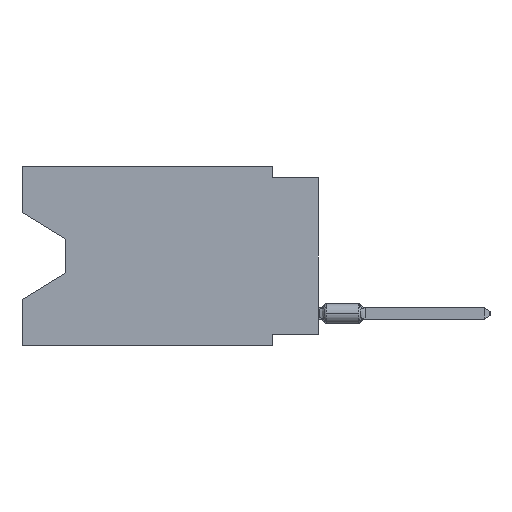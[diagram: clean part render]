
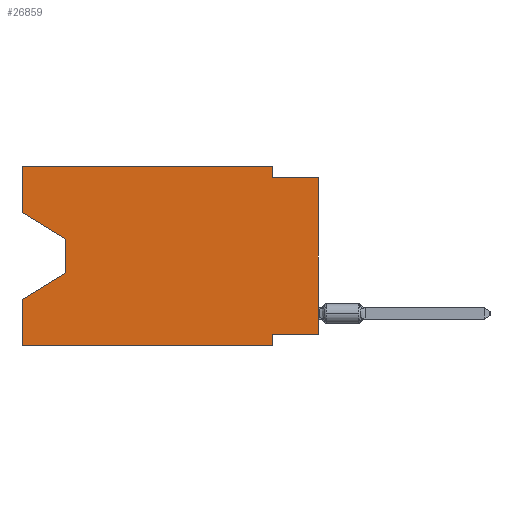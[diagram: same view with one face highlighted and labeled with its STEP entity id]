
A CAD part, left-side view. The second image highlights one B-rep face of the part: STEP entity #26859.
In plain terms, the highlighted planar face has unit normal (-1, 0, 0).
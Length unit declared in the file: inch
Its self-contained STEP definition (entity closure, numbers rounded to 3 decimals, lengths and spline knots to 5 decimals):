
#776 = CARTESIAN_POINT ( 'NONE',  ( 0., 0., -0.365 ) ) ;
#934 = LINE ( 'NONE', #68557, #21722 ) ;
#1562 = FACE_OUTER_BOUND ( 'NONE', #54318, .T. ) ;
#1840 = DIRECTION ( 'NONE',  ( 0., 0., -1. ) ) ;
#3499 = VECTOR ( 'NONE', #9635, 39.37008 ) ;
#3547 = CARTESIAN_POINT ( 'NONE',  ( 0., 0., 0. ) ) ;
#3584 = CARTESIAN_POINT ( 'NONE',  ( 0., 0., -0.025 ) ) ;
#3813 = CARTESIAN_POINT ( 'NONE',  ( 0., 0.645, 0. ) ) ;
#4023 = VECTOR ( 'NONE', #62279, 39.37008 ) ;
#4161 = CARTESIAN_POINT ( 'NONE',  ( 0., 0.1, -0.39 ) ) ;
#4468 = ORIENTED_EDGE ( 'NONE', *, *, #35396, .F. ) ;
#5954 = LINE ( 'NONE', #776, #13799 ) ;
#6317 = DIRECTION ( 'NONE',  ( 0., 1., 0. ) ) ;
#7950 = CARTESIAN_POINT ( 'NONE',  ( 0., 0.55, -0.158 ) ) ;
#8507 = ORIENTED_EDGE ( 'NONE', *, *, #49436, .F. ) ;
#9460 = CARTESIAN_POINT ( 'NONE',  ( 0., 0.1, -0.365 ) ) ;
#9635 = DIRECTION ( 'NONE',  ( 0., 0., 1. ) ) ;
#11150 = VERTEX_POINT ( 'NONE', #22287 ) ;
#11789 = ORIENTED_EDGE ( 'NONE', *, *, #65509, .F. ) ;
#13176 = ORIENTED_EDGE ( 'NONE', *, *, #52628, .F. ) ;
#13335 = PLANE ( 'NONE',  #53905 ) ;
#13682 = ORIENTED_EDGE ( 'NONE', *, *, #35279, .T. ) ;
#13693 = CARTESIAN_POINT ( 'NONE',  ( 0., 0.645, 0. ) ) ;
#13799 = VECTOR ( 'NONE', #6317, 39.37008 ) ;
#13972 = CARTESIAN_POINT ( 'NONE',  ( 0., 0.645, 0. ) ) ;
#14587 = LINE ( 'NONE', #50784, #33425 ) ;
#17159 = ORIENTED_EDGE ( 'NONE', *, *, #33899, .T. ) ;
#17227 = CARTESIAN_POINT ( 'NONE',  ( 0., 0.645, -0.28975 ) ) ;
#19438 = DIRECTION ( 'NONE',  ( 0., -0.855, -0.519 ) ) ;
#20259 = LINE ( 'NONE', #64640, #68826 ) ;
#20684 = EDGE_CURVE ( 'NONE', #61883, #63299, #20259, .T. ) ;
#21144 = EDGE_CURVE ( 'NONE', #30829, #38933, #41622, .T. ) ;
#21722 = VECTOR ( 'NONE', #52604, 39.37008 ) ;
#22186 = LINE ( 'NONE', #44742, #3499 ) ;
#22287 = CARTESIAN_POINT ( 'NONE',  ( 0., 0.1, -0.39 ) ) ;
#22472 = VECTOR ( 'NONE', #60697, 39.37008 ) ;
#23247 = DIRECTION ( 'NONE',  ( 0., 0.855, -0.519 ) ) ;
#24026 = VERTEX_POINT ( 'NONE', #34110 ) ;
#26735 = ORIENTED_EDGE ( 'NONE', *, *, #61296, .T. ) ;
#26859 = ADVANCED_FACE ( 'NONE', ( #1562 ), #13335, .F. ) ;
#28376 = CARTESIAN_POINT ( 'NONE',  ( 0., 0.645, -0.10025 ) ) ;
#29337 = LINE ( 'NONE', #51523, #4023 ) ;
#29796 = VECTOR ( 'NONE', #53049, 39.37008 ) ;
#30492 = LINE ( 'NONE', #3547, #29796 ) ;
#30829 = VERTEX_POINT ( 'NONE', #28376 ) ;
#31040 = VERTEX_POINT ( 'NONE', #33117 ) ;
#31973 = VERTEX_POINT ( 'NONE', #9460 ) ;
#32983 = ORIENTED_EDGE ( 'NONE', *, *, #20684, .F. ) ;
#33117 = CARTESIAN_POINT ( 'NONE',  ( 0., 0.645, -0.39 ) ) ;
#33425 = VECTOR ( 'NONE', #39671, 39.37008 ) ;
#33597 = CARTESIAN_POINT ( 'NONE',  ( 0., 0.55, -0.232 ) ) ;
#33899 = EDGE_CURVE ( 'NONE', #57052, #53325, #30492, .T. ) ;
#34110 = CARTESIAN_POINT ( 'NONE',  ( 0., 0.55, -0.232 ) ) ;
#35279 = EDGE_CURVE ( 'NONE', #31040, #11150, #29337, .T. ) ;
#35396 = EDGE_CURVE ( 'NONE', #63299, #53325, #934, .T. ) ;
#35742 = ORIENTED_EDGE ( 'NONE', *, *, #45989, .T. ) ;
#36021 = LINE ( 'NONE', #7950, #64969 ) ;
#37026 = VERTEX_POINT ( 'NONE', #17227 ) ;
#37175 = VECTOR ( 'NONE', #23247, 39.37008 ) ;
#38933 = VERTEX_POINT ( 'NONE', #64789 ) ;
#39671 = DIRECTION ( 'NONE',  ( 0., -1., 0. ) ) ;
#40260 = ORIENTED_EDGE ( 'NONE', *, *, #60283, .F. ) ;
#41622 = LINE ( 'NONE', #64186, #70076 ) ;
#42139 = DIRECTION ( 'NONE',  ( 1., 0., 0. ) ) ;
#44742 = CARTESIAN_POINT ( 'NONE',  ( 0., 0.645, 0. ) ) ;
#45432 = LINE ( 'NONE', #33597, #37175 ) ;
#45989 = EDGE_CURVE ( 'NONE', #38933, #24026, #36021, .T. ) ;
#48583 = DIRECTION ( 'NONE',  ( 0., 0., -1. ) ) ;
#48851 = LINE ( 'NONE', #4161, #66875 ) ;
#49386 = CARTESIAN_POINT ( 'NONE',  ( 0., 0., -0.365 ) ) ;
#49436 = EDGE_CURVE ( 'NONE', #31973, #11150, #48851, .T. ) ;
#50784 = CARTESIAN_POINT ( 'NONE',  ( 0., 0.645, 0. ) ) ;
#51523 = CARTESIAN_POINT ( 'NONE',  ( 0., 0.645, -0.39 ) ) ;
#52604 = DIRECTION ( 'NONE',  ( 0., -1., 0. ) ) ;
#52628 = EDGE_CURVE ( 'NONE', #31040, #37026, #22186, .T. ) ;
#53049 = DIRECTION ( 'NONE',  ( 0., 0., 1. ) ) ;
#53325 = VERTEX_POINT ( 'NONE', #3584 ) ;
#53905 = AXIS2_PLACEMENT_3D ( 'NONE', #13693, #42139, #63646 ) ;
#54318 = EDGE_LOOP ( 'NONE', ( #60231, #35742, #26735, #13176, #13682, #8507, #11789, #17159, #4468, #32983, #40260, #65058 ) ) ;
#57052 = VERTEX_POINT ( 'NONE', #49386 ) ;
#58882 = CARTESIAN_POINT ( 'NONE',  ( 0., 0.1, 0. ) ) ;
#58990 = CARTESIAN_POINT ( 'NONE',  ( 0., 0.1, -0.025 ) ) ;
#59964 = LINE ( 'NONE', #3813, #22472 ) ;
#60231 = ORIENTED_EDGE ( 'NONE', *, *, #21144, .T. ) ;
#60283 = EDGE_CURVE ( 'NONE', #72461, #61883, #14587, .T. ) ;
#60697 = DIRECTION ( 'NONE',  ( 0., 0., 1. ) ) ;
#61296 = EDGE_CURVE ( 'NONE', #24026, #37026, #45432, .T. ) ;
#61883 = VERTEX_POINT ( 'NONE', #58882 ) ;
#62279 = DIRECTION ( 'NONE',  ( 0., -1., 0. ) ) ;
#63299 = VERTEX_POINT ( 'NONE', #58990 ) ;
#63646 = DIRECTION ( 'NONE',  ( 0., 0., -1. ) ) ;
#64186 = CARTESIAN_POINT ( 'NONE',  ( 0., 0.645, -0.10025 ) ) ;
#64640 = CARTESIAN_POINT ( 'NONE',  ( 0., 0.1, 0. ) ) ;
#64789 = CARTESIAN_POINT ( 'NONE',  ( 0., 0.55, -0.158 ) ) ;
#64969 = VECTOR ( 'NONE', #48583, 39.37008 ) ;
#65058 = ORIENTED_EDGE ( 'NONE', *, *, #69330, .F. ) ;
#65509 = EDGE_CURVE ( 'NONE', #57052, #31973, #5954, .T. ) ;
#66875 = VECTOR ( 'NONE', #71776, 39.37008 ) ;
#68557 = CARTESIAN_POINT ( 'NONE',  ( 0., 0., -0.025 ) ) ;
#68826 = VECTOR ( 'NONE', #1840, 39.37008 ) ;
#69330 = EDGE_CURVE ( 'NONE', #30829, #72461, #59964, .T. ) ;
#70076 = VECTOR ( 'NONE', #19438, 39.37008 ) ;
#71776 = DIRECTION ( 'NONE',  ( 0., 0., -1. ) ) ;
#72461 = VERTEX_POINT ( 'NONE', #13972 ) ;
